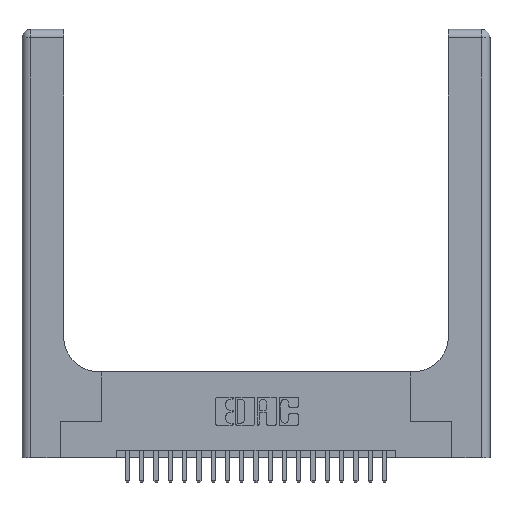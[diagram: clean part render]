
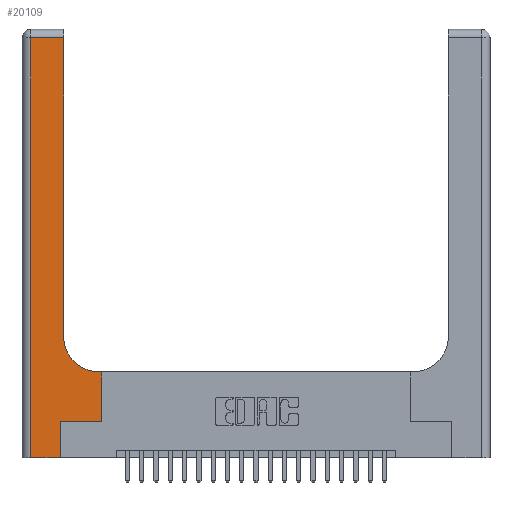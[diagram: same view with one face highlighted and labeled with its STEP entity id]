
A CAD part, top view. The second image highlights one B-rep face of the part: STEP entity #20109.
In plain terms, the highlighted planar face has unit normal (0, 0, 1).
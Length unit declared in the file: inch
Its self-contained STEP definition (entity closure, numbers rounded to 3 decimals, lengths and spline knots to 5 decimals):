
#58 = EDGE_CURVE ( 'NONE', #6954, #13222, #2407, .T. ) ;
#432 = VERTEX_POINT ( 'NONE', #10381 ) ;
#869 = VECTOR ( 'NONE', #21378, 39.37008 ) ;
#2061 = VECTOR ( 'NONE', #22385, 39.37008 ) ;
#2169 = CARTESIAN_POINT ( 'NONE',  ( 0.269, 0.25, 0.37 ) ) ;
#2407 = LINE ( 'NONE', #2169, #21003 ) ;
#2911 = DIRECTION ( 'NONE',  ( 0., 0., -1. ) ) ;
#2992 = PLANE ( 'NONE',  #12949 ) ;
#3003 = ORIENTED_EDGE ( 'NONE', *, *, #15778, .T. ) ;
#3195 = ORIENTED_EDGE ( 'NONE', *, *, #4967, .T. ) ;
#3476 = FACE_OUTER_BOUND ( 'NONE', #13519, .T. ) ;
#3938 = DIRECTION ( 'NONE',  ( 1., 0., 0. ) ) ;
#4339 = DIRECTION ( 'NONE',  ( 1., 0., 0. ) ) ;
#4680 = VERTEX_POINT ( 'NONE', #14879 ) ;
#4699 = CARTESIAN_POINT ( 'NONE',  ( 0., 3., 0.37 ) ) ;
#4967 = EDGE_CURVE ( 'NONE', #14129, #22645, #20634, .T. ) ;
#5316 = CARTESIAN_POINT ( 'NONE',  ( 0., 0., 0.37 ) ) ;
#5339 = CARTESIAN_POINT ( 'NONE',  ( 0.5585, 0.6, 0.37 ) ) ;
#5624 = DIRECTION ( 'NONE',  ( 1., 0., 0. ) ) ;
#5812 = ORIENTED_EDGE ( 'NONE', *, *, #14939, .T. ) ;
#5825 = ORIENTED_EDGE ( 'NONE', *, *, #18520, .T. ) ;
#6446 = LINE ( 'NONE', #10221, #22526 ) ;
#6495 = LINE ( 'NONE', #20041, #21471 ) ;
#6628 = LINE ( 'NONE', #14163, #9702 ) ;
#6747 = EDGE_CURVE ( 'NONE', #10449, #432, #6446, .T. ) ;
#6954 = VERTEX_POINT ( 'NONE', #17225 ) ;
#7205 = LINE ( 'NONE', #17747, #17295 ) ;
#7816 = CARTESIAN_POINT ( 'NONE',  ( 0.5415, 0.85, 0.37 ) ) ;
#7930 = CARTESIAN_POINT ( 'NONE',  ( 0.06, 0., 0.37 ) ) ;
#7966 = ORIENTED_EDGE ( 'NONE', *, *, #11310, .T. ) ;
#8670 = CARTESIAN_POINT ( 'NONE',  ( 0.2915, 3., 0.37 ) ) ;
#8702 = LINE ( 'NONE', #5316, #11509 ) ;
#9702 = VECTOR ( 'NONE', #12601, 39.37008 ) ;
#9902 = ORIENTED_EDGE ( 'NONE', *, *, #58, .T. ) ;
#10047 = VERTEX_POINT ( 'NONE', #17580 ) ;
#10077 = DIRECTION ( 'NONE',  ( -1., 0., 0. ) ) ;
#10091 = AXIS2_PLACEMENT_3D ( 'NONE', #7816, #16900, #4339 ) ;
#10221 = CARTESIAN_POINT ( 'NONE',  ( 0.2915, 0.6, 0.37 ) ) ;
#10381 = CARTESIAN_POINT ( 'NONE',  ( 0.5415, 0.6, 0.37 ) ) ;
#10449 = VERTEX_POINT ( 'NONE', #5339 ) ;
#11310 = EDGE_CURVE ( 'NONE', #13222, #10449, #6495, .T. ) ;
#11509 = VECTOR ( 'NONE', #5624, 39.37008 ) ;
#12601 = DIRECTION ( 'NONE',  ( -1., 0., 0. ) ) ;
#12882 = CARTESIAN_POINT ( 'NONE',  ( 0.06, 3., 0.37 ) ) ;
#12949 = AXIS2_PLACEMENT_3D ( 'NONE', #4699, #2911, #10077 ) ;
#13222 = VERTEX_POINT ( 'NONE', #17265 ) ;
#13455 = VERTEX_POINT ( 'NONE', #21963 ) ;
#13519 = EDGE_LOOP ( 'NONE', ( #17242, #5825, #3195, #3003, #5812, #9902, #7966, #18149, #14079 ) ) ;
#14079 = ORIENTED_EDGE ( 'NONE', *, *, #15367, .T. ) ;
#14129 = VERTEX_POINT ( 'NONE', #16456 ) ;
#14163 = CARTESIAN_POINT ( 'NONE',  ( 0., 2.94, 0.37 ) ) ;
#14879 = CARTESIAN_POINT ( 'NONE',  ( 0.2915, 2.94, 0.37 ) ) ;
#14939 = EDGE_CURVE ( 'NONE', #10047, #6954, #7205, .T. ) ;
#15367 = EDGE_CURVE ( 'NONE', #432, #13455, #18816, .T. ) ;
#15778 = EDGE_CURVE ( 'NONE', #22645, #10047, #8702, .T. ) ;
#16353 = LINE ( 'NONE', #8670, #869 ) ;
#16456 = CARTESIAN_POINT ( 'NONE',  ( 0.06, 2.94, 0.37 ) ) ;
#16900 = DIRECTION ( 'NONE',  ( 0., 0., -1. ) ) ;
#17225 = CARTESIAN_POINT ( 'NONE',  ( 0.269, 0.25, 0.37 ) ) ;
#17242 = ORIENTED_EDGE ( 'NONE', *, *, #22235, .T. ) ;
#17265 = CARTESIAN_POINT ( 'NONE',  ( 0.5585, 0.25, 0.37 ) ) ;
#17295 = VECTOR ( 'NONE', #17594, 39.37008 ) ;
#17580 = CARTESIAN_POINT ( 'NONE',  ( 0.269, 0., 0.37 ) ) ;
#17594 = DIRECTION ( 'NONE',  ( 0., 1., 0. ) ) ;
#17747 = CARTESIAN_POINT ( 'NONE',  ( 0.269, 0., 0.37 ) ) ;
#18149 = ORIENTED_EDGE ( 'NONE', *, *, #6747, .T. ) ;
#18520 = EDGE_CURVE ( 'NONE', #4680, #14129, #6628, .T. ) ;
#18816 = CIRCLE ( 'NONE', #10091, 0.25 ) ;
#20041 = CARTESIAN_POINT ( 'NONE',  ( 0.5585, 0.25, 0.37 ) ) ;
#20109 = ADVANCED_FACE ( 'NONE', ( #3476 ), #2992, .F. ) ;
#20634 = LINE ( 'NONE', #12882, #2061 ) ;
#21003 = VECTOR ( 'NONE', #3938, 39.37008 ) ;
#21378 = DIRECTION ( 'NONE',  ( 0., 1., 0. ) ) ;
#21471 = VECTOR ( 'NONE', #21665, 39.37008 ) ;
#21665 = DIRECTION ( 'NONE',  ( 0., 1., 0. ) ) ;
#21963 = CARTESIAN_POINT ( 'NONE',  ( 0.2915, 0.85, 0.37 ) ) ;
#22235 = EDGE_CURVE ( 'NONE', #13455, #4680, #16353, .T. ) ;
#22385 = DIRECTION ( 'NONE',  ( 0., -1., 0. ) ) ;
#22508 = DIRECTION ( 'NONE',  ( -1., 0., 0. ) ) ;
#22526 = VECTOR ( 'NONE', #22508, 39.37008 ) ;
#22645 = VERTEX_POINT ( 'NONE', #7930 ) ;
